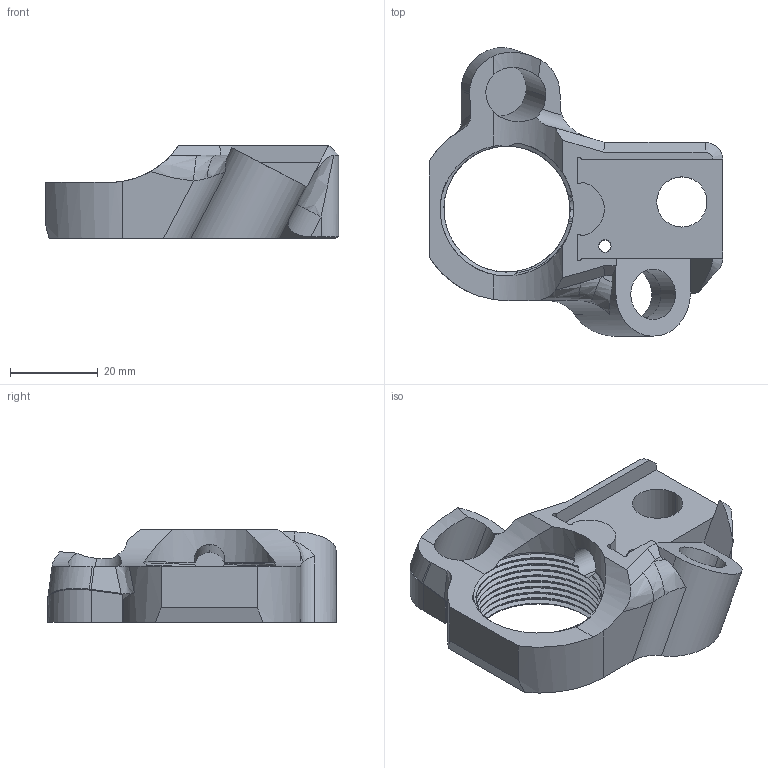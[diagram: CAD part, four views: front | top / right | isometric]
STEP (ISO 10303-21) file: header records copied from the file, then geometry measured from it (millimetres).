
FILE_DESCRIPTION (( 'STEP AP203' ), '1' );
FILE_NAME ('AF-HF-LR-PRT-002-STEP.STEP', '2020-11-01T12:16:52', ( '' ), ( '' ), 'SwSTEP 2.0', 'SolidWorks 2018', '' );
FILE_SCHEMA (( 'CONFIG_CONTROL_DESIGN' ));
Length unit declared in the file: inch
Products named in the file (1): AF-HF-LR-PRT-002-STEP
Bounding box: 66.83 x 65.69 x 21.17 mm (x, y, z)
Volume: 26899.1 mm3; surface area: 13382.9 mm2
Topology: 1 solids, 1 shells, 149 faces, 416 edges, 270 vertices
Faces by surface type: cylinder 59, plane 53, bspline 21, cone 16
Entity records: 9206 total; most frequent: CARTESIAN_POINT 5660, ORIENTED_EDGE 826, DIRECTION 615, EDGE_CURVE 413, VERTEX_POINT 269, AXIS2_PLACEMENT_3D 217, VECTOR 181, LINE 181
